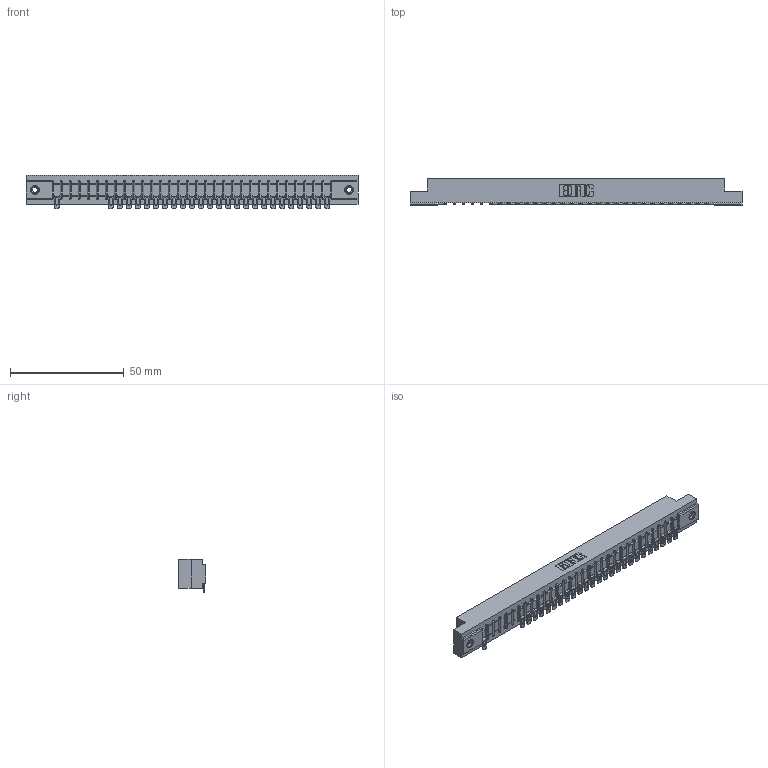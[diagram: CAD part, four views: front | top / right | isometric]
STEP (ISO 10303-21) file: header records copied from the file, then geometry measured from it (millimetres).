
FILE_DESCRIPTION (( 'STEP AP203' ), '1' );
FILE_NAME ('357-031-554-108.STEP', '2018-08-09T22:53:11', ( '' ), ( '' ), 'SwSTEP 2.0', 'SolidWorks 2016', '' );
FILE_SCHEMA (( 'CONFIG_CONTROL_DESIGN' ));
Length unit declared in the file: inch
Products named in the file (4): 307 Part_.156 Dia Mounting Holes; 307-290-002_554; 345-250-001_345-250-003-102; 357-031-554-108
Assembly tree (29 placements, depth 2):
  357-031-554-108
    307 Part_.156 Dia Mounting Holes
    307-290-002_554  x26
    345-250-001_345-250-003-102  x2
Bounding box: 145.85 x 12.01 x 14.52 mm (x, y, z)
Volume: 15383.6 mm3; surface area: 18294.9 mm2
Topology: 29 solids, 29 shells, 2416 faces, 7357 edges, 4810 vertices
Faces by surface type: plane 1358, cylinder 978, sphere 64, cone 12, torus 4
Entity records: 29922 total; most frequent: CARTESIAN_POINT 5048, ORIENTED_EDGE 5036, DIRECTION 4920, EDGE_CURVE 2518, LINE 1916, VECTOR 1916, VERTEX_POINT 1630, AXIS2_PLACEMENT_3D 1502
